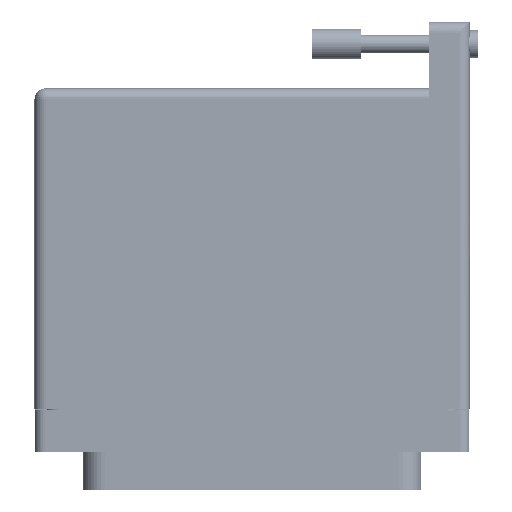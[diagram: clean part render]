
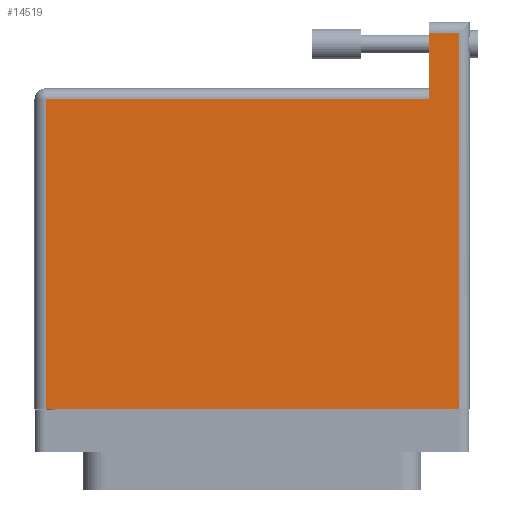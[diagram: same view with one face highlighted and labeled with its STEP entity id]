
A CAD part, front view. The second image highlights one B-rep face of the part: STEP entity #14519.
In plain terms, the highlighted face is planar.
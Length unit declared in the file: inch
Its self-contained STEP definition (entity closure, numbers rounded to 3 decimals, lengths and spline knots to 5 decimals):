
#2255 = CARTESIAN_POINT ( 'NONE',  ( -1.3775, 2.28, 0.765 ) ) ;
#2295 = ORIENTED_EDGE ( 'NONE', *, *, #59960, .T. ) ;
#2977 = LINE ( 'NONE', #42918, #87111 ) ;
#3981 = CARTESIAN_POINT ( 'NONE',  ( -1.3775, 1.93, 0.765 ) ) ;
#5559 = CARTESIAN_POINT ( 'NONE',  ( -1.3775, 1.86, 0.765 ) ) ;
#7602 = VERTEX_POINT ( 'NONE', #59644 ) ;
#12192 = CARTESIAN_POINT ( 'NONE',  ( 1.1215, 1.86, 0.765 ) ) ;
#13298 = FACE_OUTER_BOUND ( 'NONE', #30935, .T. ) ;
#14519 = ADVANCED_FACE ( 'NONE', ( #13298 ), #44420, .F. ) ;
#14759 = EDGE_CURVE ( 'NONE', #19008, #20814, #20818, .T. ) ;
#15115 = VERTEX_POINT ( 'NONE', #51292 ) ;
#16310 = AXIS2_PLACEMENT_3D ( 'NONE', #3981, #58842, #79048 ) ;
#19008 = VERTEX_POINT ( 'NONE', #45573 ) ;
#20814 = VERTEX_POINT ( 'NONE', #66536 ) ;
#20818 = LINE ( 'NONE', #23172, #73662 ) ;
#23172 = CARTESIAN_POINT ( 'NONE',  ( 1.3075, 2.35, 0.765 ) ) ;
#23545 = VERTEX_POINT ( 'NONE', #33233 ) ;
#28452 = DIRECTION ( 'NONE',  ( 1., 0., 0. ) ) ;
#30935 = EDGE_LOOP ( 'NONE', ( #72145, #54918, #2295, #32396, #58310, #65115 ) ) ;
#32396 = ORIENTED_EDGE ( 'NONE', *, *, #76352, .T. ) ;
#33233 = CARTESIAN_POINT ( 'NONE',  ( 1.1215, 2.28, 0.765 ) ) ;
#33486 = CARTESIAN_POINT ( 'NONE',  ( -1.3075, -0.1, 0.765 ) ) ;
#39234 = VERTEX_POINT ( 'NONE', #12192 ) ;
#42918 = CARTESIAN_POINT ( 'NONE',  ( -1.3775, -0.1, 0.765 ) ) ;
#43271 = DIRECTION ( 'NONE',  ( -1., 0., 0. ) ) ;
#44420 = PLANE ( 'NONE',  #16310 ) ;
#45573 = CARTESIAN_POINT ( 'NONE',  ( 1.3075, -0.1, 0.765 ) ) ;
#46913 = LINE ( 'NONE', #2255, #59890 ) ;
#47098 = DIRECTION ( 'NONE',  ( 0., -1., 0. ) ) ;
#48022 = VECTOR ( 'NONE', #47098, 39.37008 ) ;
#49066 = LINE ( 'NONE', #33486, #48022 ) ;
#49218 = LINE ( 'NONE', #5559, #54606 ) ;
#50645 = EDGE_CURVE ( 'NONE', #23545, #39234, #63537, .T. ) ;
#51292 = CARTESIAN_POINT ( 'NONE',  ( -1.3075, -0.1, 0.765 ) ) ;
#51740 = CARTESIAN_POINT ( 'NONE',  ( 1.1215, 2.35, 0.765 ) ) ;
#54606 = VECTOR ( 'NONE', #80580, 39.37008 ) ;
#54918 = ORIENTED_EDGE ( 'NONE', *, *, #59568, .T. ) ;
#58310 = ORIENTED_EDGE ( 'NONE', *, *, #14759, .T. ) ;
#58842 = DIRECTION ( 'NONE',  ( 0., 0., -1. ) ) ;
#59568 = EDGE_CURVE ( 'NONE', #39234, #7602, #49218, .T. ) ;
#59644 = CARTESIAN_POINT ( 'NONE',  ( -1.3075, 1.86, 0.765 ) ) ;
#59890 = VECTOR ( 'NONE', #43271, 39.37008 ) ;
#59960 = EDGE_CURVE ( 'NONE', #7602, #15115, #49066, .T. ) ;
#63537 = LINE ( 'NONE', #51740, #87339 ) ;
#65115 = ORIENTED_EDGE ( 'NONE', *, *, #67231, .T. ) ;
#66536 = CARTESIAN_POINT ( 'NONE',  ( 1.3075, 2.28, 0.765 ) ) ;
#67231 = EDGE_CURVE ( 'NONE', #20814, #23545, #46913, .T. ) ;
#71424 = DIRECTION ( 'NONE',  ( 0., 1., 0. ) ) ;
#72145 = ORIENTED_EDGE ( 'NONE', *, *, #50645, .T. ) ;
#72523 = DIRECTION ( 'NONE',  ( 0., -1., 0. ) ) ;
#73662 = VECTOR ( 'NONE', #71424, 39.37008 ) ;
#76352 = EDGE_CURVE ( 'NONE', #15115, #19008, #2977, .T. ) ;
#79048 = DIRECTION ( 'NONE',  ( -1., 0., 0. ) ) ;
#80580 = DIRECTION ( 'NONE',  ( -1., 0., 0. ) ) ;
#87111 = VECTOR ( 'NONE', #28452, 39.37008 ) ;
#87339 = VECTOR ( 'NONE', #72523, 39.37008 ) ;
